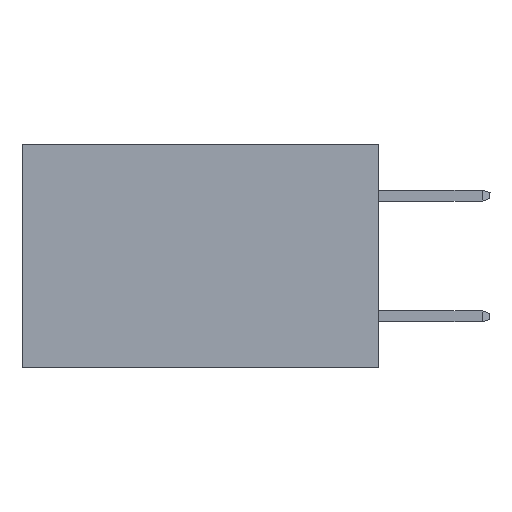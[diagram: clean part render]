
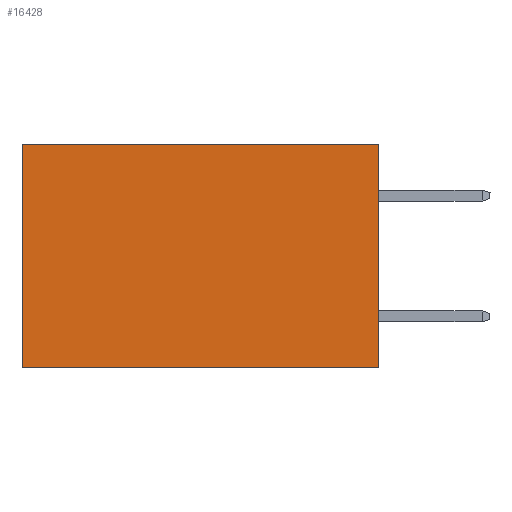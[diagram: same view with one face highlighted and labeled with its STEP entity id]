
A CAD part, left-side view. The second image highlights one B-rep face of the part: STEP entity #16428.
In plain terms, the highlighted planar face has unit normal (-1, 0, 0).
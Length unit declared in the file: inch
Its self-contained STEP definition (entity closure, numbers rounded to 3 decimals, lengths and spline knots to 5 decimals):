
#771 = EDGE_CURVE ( 'NONE', #8784, #8665, #14533, .T. ) ;
#1958 = CARTESIAN_POINT ( 'NONE',  ( 0.277, 0., -0.37 ) ) ;
#2361 = LINE ( 'NONE', #16889, #5780 ) ;
#2703 = ORIENTED_EDGE ( 'NONE', *, *, #771, .T. ) ;
#2798 = CARTESIAN_POINT ( 'NONE',  ( 0.277, 0., -0.37 ) ) ;
#2904 = LINE ( 'NONE', #16680, #13134 ) ;
#3848 = DIRECTION ( 'NONE',  ( 0., 1., 0. ) ) ;
#4126 = EDGE_CURVE ( 'NONE', #14959, #8665, #17915, .T. ) ;
#4799 = CARTESIAN_POINT ( 'NONE',  ( 0.277, 0.59, -0.37 ) ) ;
#5780 = VECTOR ( 'NONE', #12751, 39.37008 ) ;
#5944 = DIRECTION ( 'NONE',  ( 1., 0., 0. ) ) ;
#7335 = VERTEX_POINT ( 'NONE', #8205 ) ;
#8075 = CARTESIAN_POINT ( 'NONE',  ( 0.277, 0.59, -0.37 ) ) ;
#8205 = CARTESIAN_POINT ( 'NONE',  ( 0.277, 0., 0. ) ) ;
#8665 = VERTEX_POINT ( 'NONE', #8075 ) ;
#8784 = VERTEX_POINT ( 'NONE', #11175 ) ;
#9208 = ORIENTED_EDGE ( 'NONE', *, *, #11453, .T. ) ;
#9524 = ORIENTED_EDGE ( 'NONE', *, *, #4126, .F. ) ;
#9606 = EDGE_LOOP ( 'NONE', ( #2703, #9524, #10660, #9208 ) ) ;
#10271 = VECTOR ( 'NONE', #15306, 39.37008 ) ;
#10660 = ORIENTED_EDGE ( 'NONE', *, *, #14372, .F. ) ;
#10708 = FACE_OUTER_BOUND ( 'NONE', #9606, .T. ) ;
#11175 = CARTESIAN_POINT ( 'NONE',  ( 0.277, 0.59, 0. ) ) ;
#11453 = EDGE_CURVE ( 'NONE', #7335, #8784, #2904, .T. ) ;
#12751 = DIRECTION ( 'NONE',  ( 0., 0., -1. ) ) ;
#12872 = DIRECTION ( 'NONE',  ( 0., 1., 0. ) ) ;
#13134 = VECTOR ( 'NONE', #3848, 39.37008 ) ;
#13659 = AXIS2_PLACEMENT_3D ( 'NONE', #14562, #5944, #15971 ) ;
#14223 = VECTOR ( 'NONE', #12872, 39.37008 ) ;
#14372 = EDGE_CURVE ( 'NONE', #7335, #14959, #2361, .T. ) ;
#14533 = LINE ( 'NONE', #4799, #10271 ) ;
#14562 = CARTESIAN_POINT ( 'NONE',  ( 0.277, 0., -0.37 ) ) ;
#14959 = VERTEX_POINT ( 'NONE', #2798 ) ;
#15306 = DIRECTION ( 'NONE',  ( 0., 0., -1. ) ) ;
#15913 = PLANE ( 'NONE',  #13659 ) ;
#15971 = DIRECTION ( 'NONE',  ( 0., 0., -1. ) ) ;
#16428 = ADVANCED_FACE ( 'NONE', ( #10708 ), #15913, .F. ) ;
#16680 = CARTESIAN_POINT ( 'NONE',  ( 0.277, 0., 0. ) ) ;
#16889 = CARTESIAN_POINT ( 'NONE',  ( 0.277, 0., -0.37 ) ) ;
#17915 = LINE ( 'NONE', #1958, #14223 ) ;
